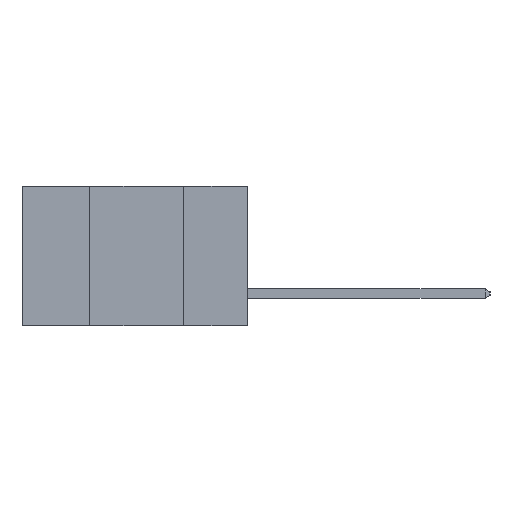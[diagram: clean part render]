
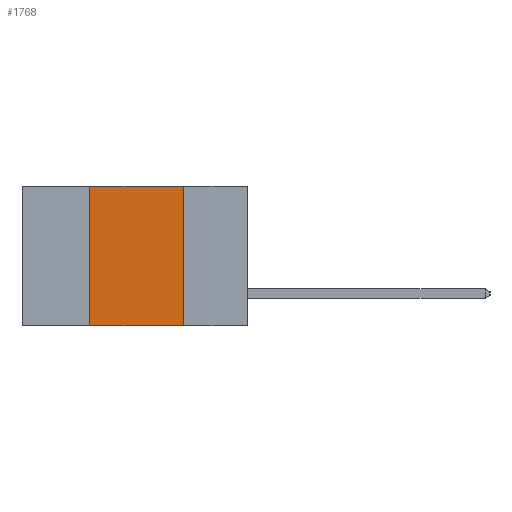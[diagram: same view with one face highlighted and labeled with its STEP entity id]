
A CAD part, left-side view. The second image highlights one B-rep face of the part: STEP entity #1768.
In plain terms, the highlighted planar face has unit normal (-1, 0, 0).
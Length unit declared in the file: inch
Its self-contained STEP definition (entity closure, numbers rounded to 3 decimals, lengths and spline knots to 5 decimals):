
#393 = VERTEX_POINT ( 'NONE', #2009 ) ;
#430 = CARTESIAN_POINT ( 'NONE',  ( 0., 0.17, 0. ) ) ;
#665 = EDGE_CURVE ( 'NONE', #2325, #8546, #4994, .T. ) ;
#1205 = CARTESIAN_POINT ( 'NONE',  ( 0., 0.6, 0. ) ) ;
#1483 = DIRECTION ( 'NONE',  ( 0., -1., 0. ) ) ;
#1768 = ADVANCED_FACE ( 'NONE', ( #7487 ), #5210, .F. ) ;
#2009 = CARTESIAN_POINT ( 'NONE',  ( 0., 0.17, -0.37 ) ) ;
#2232 = ORIENTED_EDGE ( 'NONE', *, *, #7698, .T. ) ;
#2325 = VERTEX_POINT ( 'NONE', #7030 ) ;
#2569 = DIRECTION ( 'NONE',  ( 0., 0., -1. ) ) ;
#2799 = EDGE_LOOP ( 'NONE', ( #5070, #3247, #4247, #2232 ) ) ;
#2950 = VERTEX_POINT ( 'NONE', #5550 ) ;
#3069 = DIRECTION ( 'NONE',  ( 0., 0., 1. ) ) ;
#3124 = VECTOR ( 'NONE', #2569, 39.37008 ) ;
#3131 = CARTESIAN_POINT ( 'NONE',  ( 0., 0.42, 0. ) ) ;
#3247 = ORIENTED_EDGE ( 'NONE', *, *, #665, .F. ) ;
#3297 = CARTESIAN_POINT ( 'NONE',  ( 0., 0.6, 0. ) ) ;
#4247 = ORIENTED_EDGE ( 'NONE', *, *, #8245, .F. ) ;
#4587 = EDGE_CURVE ( 'NONE', #8546, #393, #7153, .T. ) ;
#4815 = DIRECTION ( 'NONE',  ( 1., 0., 0. ) ) ;
#4994 = LINE ( 'NONE', #1205, #8363 ) ;
#5070 = ORIENTED_EDGE ( 'NONE', *, *, #4587, .F. ) ;
#5210 = PLANE ( 'NONE',  #6802 ) ;
#5550 = CARTESIAN_POINT ( 'NONE',  ( 0., 0.42, -0.37 ) ) ;
#5630 = VECTOR ( 'NONE', #7075, 39.37008 ) ;
#6296 = VECTOR ( 'NONE', #3069, 39.37008 ) ;
#6802 = AXIS2_PLACEMENT_3D ( 'NONE', #3297, #4815, #8729 ) ;
#7030 = CARTESIAN_POINT ( 'NONE',  ( 0., 0.42, 0. ) ) ;
#7075 = DIRECTION ( 'NONE',  ( 0., -1., 0. ) ) ;
#7135 = CARTESIAN_POINT ( 'NONE',  ( 0., 0.17, 0. ) ) ;
#7153 = LINE ( 'NONE', #430, #3124 ) ;
#7400 = LINE ( 'NONE', #8255, #5630 ) ;
#7487 = FACE_OUTER_BOUND ( 'NONE', #2799, .T. ) ;
#7698 = EDGE_CURVE ( 'NONE', #2950, #393, #7400, .T. ) ;
#7812 = LINE ( 'NONE', #3131, #6296 ) ;
#8245 = EDGE_CURVE ( 'NONE', #2950, #2325, #7812, .T. ) ;
#8255 = CARTESIAN_POINT ( 'NONE',  ( 0., 0.6, -0.37 ) ) ;
#8363 = VECTOR ( 'NONE', #1483, 39.37008 ) ;
#8546 = VERTEX_POINT ( 'NONE', #7135 ) ;
#8729 = DIRECTION ( 'NONE',  ( 0., 0., -1. ) ) ;
